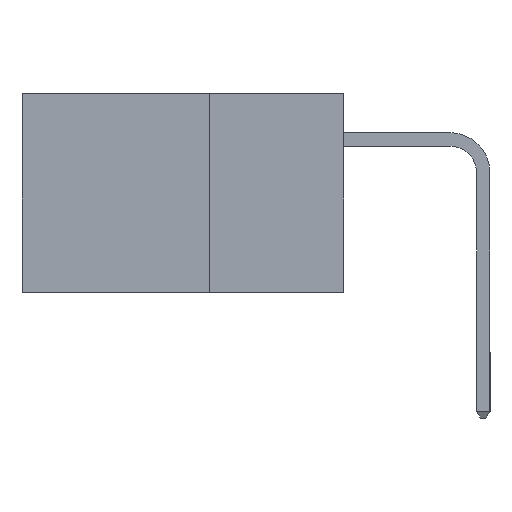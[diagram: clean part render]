
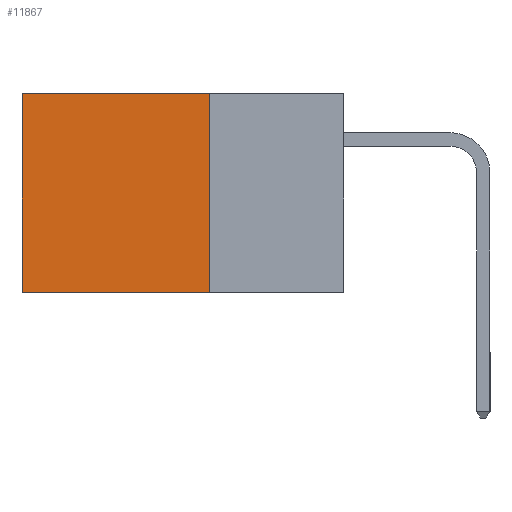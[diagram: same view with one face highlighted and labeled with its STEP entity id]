
A CAD part, left-side view. The second image highlights one B-rep face of the part: STEP entity #11867.
In plain terms, the highlighted planar face has unit normal (-1, 0, 0).
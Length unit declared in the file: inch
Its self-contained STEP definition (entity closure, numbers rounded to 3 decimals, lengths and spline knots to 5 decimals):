
#67 = ORIENTED_EDGE ( 'NONE', *, *, #11353, .T. ) ;
#295 = LINE ( 'NONE', #24982, #19988 ) ;
#335 = CARTESIAN_POINT ( 'NONE',  ( 0.2615, 0.6, 0. ) ) ;
#463 = ORIENTED_EDGE ( 'NONE', *, *, #25522, .F. ) ;
#847 = VECTOR ( 'NONE', #14646, 39.37008 ) ;
#1194 = EDGE_CURVE ( 'NONE', #21714, #19797, #15179, .T. ) ;
#2378 = PLANE ( 'NONE',  #5147 ) ;
#2507 = FACE_OUTER_BOUND ( 'NONE', #5207, .T. ) ;
#2767 = VECTOR ( 'NONE', #21427, 39.37008 ) ;
#2931 = DIRECTION ( 'NONE',  ( 0., 0., -1. ) ) ;
#5073 = VECTOR ( 'NONE', #14957, 39.37008 ) ;
#5147 = AXIS2_PLACEMENT_3D ( 'NONE', #22845, #18853, #20478 ) ;
#5184 = ORIENTED_EDGE ( 'NONE', *, *, #18974, .T. ) ;
#5207 = EDGE_LOOP ( 'NONE', ( #67, #463, #16126, #5184 ) ) ;
#5237 = CARTESIAN_POINT ( 'NONE',  ( 0.2615, 0.6, -0.37 ) ) ;
#7932 = VERTEX_POINT ( 'NONE', #335 ) ;
#9104 = CARTESIAN_POINT ( 'NONE',  ( 0.2615, 0.25, -0.37 ) ) ;
#9323 = VERTEX_POINT ( 'NONE', #5237 ) ;
#10762 = CARTESIAN_POINT ( 'NONE',  ( 0.2615, 0.25, 0. ) ) ;
#11353 = EDGE_CURVE ( 'NONE', #7932, #9323, #295, .T. ) ;
#11867 = ADVANCED_FACE ( 'NONE', ( #2507 ), #2378, .F. ) ;
#13188 = CARTESIAN_POINT ( 'NONE',  ( 0.2615, 0.25, 0. ) ) ;
#14646 = DIRECTION ( 'NONE',  ( 0., 0., -1. ) ) ;
#14957 = DIRECTION ( 'NONE',  ( 0., 1., 0. ) ) ;
#15179 = LINE ( 'NONE', #16768, #847 ) ;
#15314 = LINE ( 'NONE', #13188, #2767 ) ;
#16126 = ORIENTED_EDGE ( 'NONE', *, *, #1194, .F. ) ;
#16768 = CARTESIAN_POINT ( 'NONE',  ( 0.2615, 0.25, -0.37 ) ) ;
#18400 = CARTESIAN_POINT ( 'NONE',  ( 0.2615, 0.25, -0.37 ) ) ;
#18853 = DIRECTION ( 'NONE',  ( 1., 0., 0. ) ) ;
#18974 = EDGE_CURVE ( 'NONE', #21714, #7932, #15314, .T. ) ;
#19797 = VERTEX_POINT ( 'NONE', #18400 ) ;
#19988 = VECTOR ( 'NONE', #2931, 39.37008 ) ;
#20478 = DIRECTION ( 'NONE',  ( 0., 0., -1. ) ) ;
#21075 = LINE ( 'NONE', #9104, #5073 ) ;
#21427 = DIRECTION ( 'NONE',  ( 0., 1., 0. ) ) ;
#21714 = VERTEX_POINT ( 'NONE', #10762 ) ;
#22845 = CARTESIAN_POINT ( 'NONE',  ( 0.2615, 0.25, -0.37 ) ) ;
#24982 = CARTESIAN_POINT ( 'NONE',  ( 0.2615, 0.6, -0.37 ) ) ;
#25522 = EDGE_CURVE ( 'NONE', #19797, #9323, #21075, .T. ) ;
